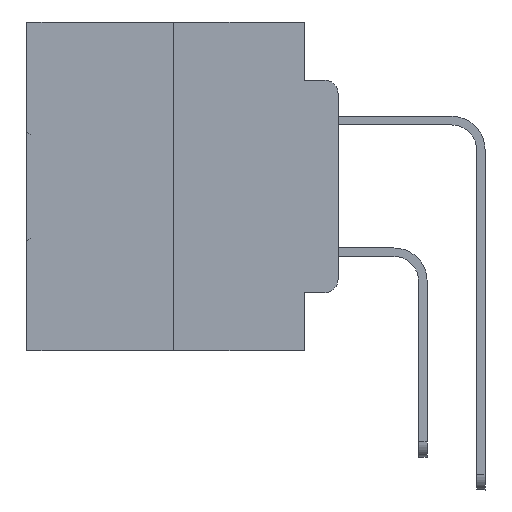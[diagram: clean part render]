
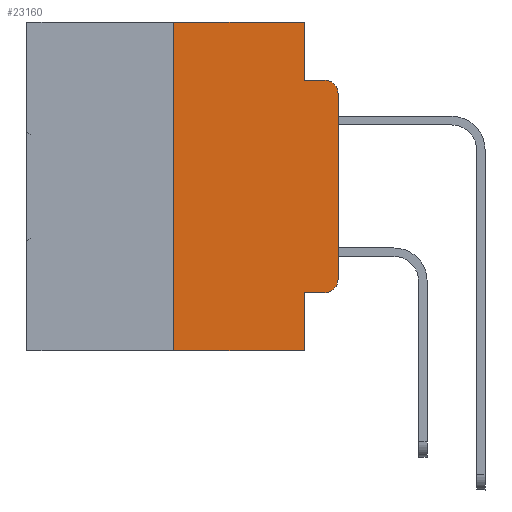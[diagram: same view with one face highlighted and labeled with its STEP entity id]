
A CAD part, left-side view. The second image highlights one B-rep face of the part: STEP entity #23160.
In plain terms, the highlighted planar face has unit normal (-1, 0, 0).
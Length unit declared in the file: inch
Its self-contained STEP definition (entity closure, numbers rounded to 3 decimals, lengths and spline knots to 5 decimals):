
#337 = DIRECTION ( 'NONE',  ( 0., -1., 0. ) ) ;
#533 = DIRECTION ( 'NONE',  ( 0., 0., -1. ) ) ;
#1106 = PLANE ( 'NONE',  #16063 ) ;
#1259 = CARTESIAN_POINT ( 'NONE',  ( 0., 0.02, -0.4115 ) ) ;
#2069 = VERTEX_POINT ( 'NONE', #13493 ) ;
#2767 = LINE ( 'NONE', #33832, #28001 ) ;
#3178 = VECTOR ( 'NONE', #30919, 39.37008 ) ;
#4214 = ORIENTED_EDGE ( 'NONE', *, *, #30660, .F. ) ;
#4681 = DIRECTION ( 'NONE',  ( 0., 0., -1. ) ) ;
#4715 = ORIENTED_EDGE ( 'NONE', *, *, #10236, .T. ) ;
#5034 = VERTEX_POINT ( 'NONE', #24503 ) ;
#5288 = EDGE_CURVE ( 'NONE', #18608, #2069, #23830, .T. ) ;
#5909 = DIRECTION ( 'NONE',  ( -1., 0., 0. ) ) ;
#5970 = ORIENTED_EDGE ( 'NONE', *, *, #7502, .T. ) ;
#6128 = DIRECTION ( 'NONE',  ( 0., -1., 0. ) ) ;
#7029 = EDGE_CURVE ( 'NONE', #17419, #32176, #28485, .T. ) ;
#7287 = LINE ( 'NONE', #23241, #27819 ) ;
#7332 = DIRECTION ( 'NONE',  ( 0., 0., 1. ) ) ;
#7502 = EDGE_CURVE ( 'NONE', #32616, #20159, #28681, .T. ) ;
#7705 = EDGE_CURVE ( 'NONE', #13952, #5034, #17407, .T. ) ;
#8646 = CARTESIAN_POINT ( 'NONE',  ( 0., 0., -0.1085 ) ) ;
#10236 = EDGE_CURVE ( 'NONE', #32176, #32616, #24998, .T. ) ;
#10920 = DIRECTION ( 'NONE',  ( 0., 0., -1. ) ) ;
#11332 = CARTESIAN_POINT ( 'NONE',  ( 0., 0.473, 0. ) ) ;
#11667 = DIRECTION ( 'NONE',  ( 0., 0., -1. ) ) ;
#11703 = AXIS2_PLACEMENT_3D ( 'NONE', #29291, #5909, #533 ) ;
#11848 = VECTOR ( 'NONE', #7332, 39.37008 ) ;
#12761 = CARTESIAN_POINT ( 'NONE',  ( 0., 0., -0.3915 ) ) ;
#13493 = CARTESIAN_POINT ( 'NONE',  ( 0., 0.051, -0.5 ) ) ;
#13754 = DIRECTION ( 'NONE',  ( 1., 0., 0. ) ) ;
#13788 = CARTESIAN_POINT ( 'NONE',  ( 0., 0.02, -0.1085 ) ) ;
#13952 = VERTEX_POINT ( 'NONE', #18247 ) ;
#13972 = VECTOR ( 'NONE', #337, 39.37008 ) ;
#14145 = DIRECTION ( 'NONE',  ( -1., 0., 0. ) ) ;
#14207 = LINE ( 'NONE', #30127, #13972 ) ;
#14226 = VERTEX_POINT ( 'NONE', #22384 ) ;
#15328 = DIRECTION ( 'NONE',  ( 0., -1., 0. ) ) ;
#15334 = VECTOR ( 'NONE', #31271, 39.37008 ) ;
#15493 = CARTESIAN_POINT ( 'NONE',  ( 0., 0.051, -0.4115 ) ) ;
#16063 = AXIS2_PLACEMENT_3D ( 'NONE', #11332, #13754, #11667 ) ;
#16099 = AXIS2_PLACEMENT_3D ( 'NONE', #13788, #14145, #19527 ) ;
#16433 = EDGE_CURVE ( 'NONE', #18608, #14226, #27969, .T. ) ;
#17311 = ORIENTED_EDGE ( 'NONE', *, *, #27454, .F. ) ;
#17407 = LINE ( 'NONE', #19839, #24846 ) ;
#17419 = VERTEX_POINT ( 'NONE', #18523 ) ;
#18247 = CARTESIAN_POINT ( 'NONE',  ( 0., 0.051, -0.0885 ) ) ;
#18523 = CARTESIAN_POINT ( 'NONE',  ( 0., 0.051, -0.4115 ) ) ;
#18608 = VERTEX_POINT ( 'NONE', #33471 ) ;
#19156 = FACE_OUTER_BOUND ( 'NONE', #20381, .T. ) ;
#19527 = DIRECTION ( 'NONE',  ( 0., 0., -1. ) ) ;
#19839 = CARTESIAN_POINT ( 'NONE',  ( 0., 0.051, -0.0885 ) ) ;
#20159 = VERTEX_POINT ( 'NONE', #8646 ) ;
#20381 = EDGE_LOOP ( 'NONE', ( #5970, #23599, #24980, #4214, #17311, #33792, #25172, #31359, #32713, #4715 ) ) ;
#20553 = CARTESIAN_POINT ( 'NONE',  ( 0., 0.473, -0.5 ) ) ;
#20785 = CARTESIAN_POINT ( 'NONE',  ( 0., 0.051, 0. ) ) ;
#21508 = VECTOR ( 'NONE', #15328, 39.37008 ) ;
#22384 = CARTESIAN_POINT ( 'NONE',  ( 0., 0.25, 0. ) ) ;
#23160 = ADVANCED_FACE ( 'NONE', ( #19156 ), #1106, .F. ) ;
#23241 = CARTESIAN_POINT ( 'NONE',  ( 0., 0.051, 0. ) ) ;
#23599 = ORIENTED_EDGE ( 'NONE', *, *, #32997, .T. ) ;
#23830 = LINE ( 'NONE', #20553, #15334 ) ;
#24503 = CARTESIAN_POINT ( 'NONE',  ( 0., 0.02, -0.0885 ) ) ;
#24846 = VECTOR ( 'NONE', #6128, 39.37008 ) ;
#24953 = CIRCLE ( 'NONE', #16099, 0.02 ) ;
#24980 = ORIENTED_EDGE ( 'NONE', *, *, #7705, .F. ) ;
#24998 = CIRCLE ( 'NONE', #11703, 0.02 ) ;
#25172 = ORIENTED_EDGE ( 'NONE', *, *, #5288, .T. ) ;
#25576 = VERTEX_POINT ( 'NONE', #20785 ) ;
#27270 = EDGE_CURVE ( 'NONE', #17419, #2069, #7287, .T. ) ;
#27454 = EDGE_CURVE ( 'NONE', #14226, #25576, #14207, .T. ) ;
#27819 = VECTOR ( 'NONE', #4681, 39.37008 ) ;
#27969 = LINE ( 'NONE', #31227, #11848 ) ;
#28001 = VECTOR ( 'NONE', #10920, 39.37008 ) ;
#28485 = LINE ( 'NONE', #15493, #21508 ) ;
#28681 = LINE ( 'NONE', #33689, #3178 ) ;
#29291 = CARTESIAN_POINT ( 'NONE',  ( 0., 0.02, -0.3915 ) ) ;
#30127 = CARTESIAN_POINT ( 'NONE',  ( 0., 0.473, 0. ) ) ;
#30660 = EDGE_CURVE ( 'NONE', #25576, #13952, #2767, .T. ) ;
#30919 = DIRECTION ( 'NONE',  ( 0., 0., 1. ) ) ;
#31227 = CARTESIAN_POINT ( 'NONE',  ( 0., 0.25, 0. ) ) ;
#31271 = DIRECTION ( 'NONE',  ( 0., -1., 0. ) ) ;
#31359 = ORIENTED_EDGE ( 'NONE', *, *, #27270, .F. ) ;
#32176 = VERTEX_POINT ( 'NONE', #1259 ) ;
#32616 = VERTEX_POINT ( 'NONE', #12761 ) ;
#32713 = ORIENTED_EDGE ( 'NONE', *, *, #7029, .T. ) ;
#32997 = EDGE_CURVE ( 'NONE', #20159, #5034, #24953, .T. ) ;
#33471 = CARTESIAN_POINT ( 'NONE',  ( 0., 0.25, -0.5 ) ) ;
#33689 = CARTESIAN_POINT ( 'NONE',  ( 0., 0., 0. ) ) ;
#33792 = ORIENTED_EDGE ( 'NONE', *, *, #16433, .F. ) ;
#33832 = CARTESIAN_POINT ( 'NONE',  ( 0., 0.051, 0. ) ) ;
